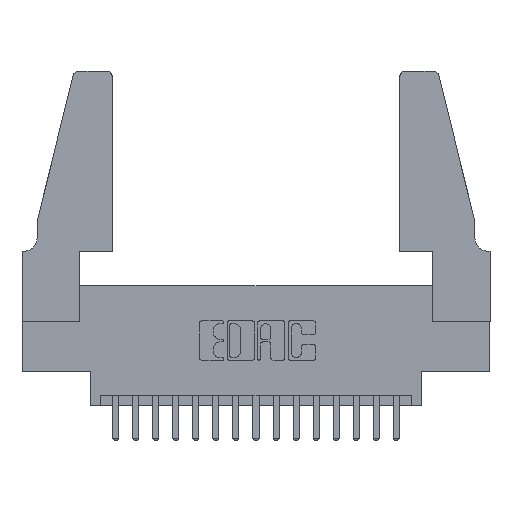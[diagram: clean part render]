
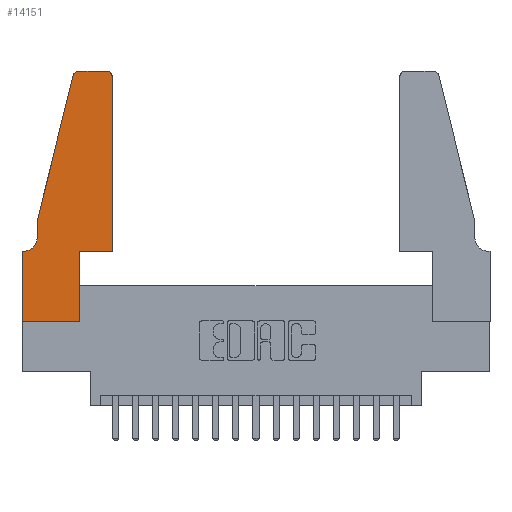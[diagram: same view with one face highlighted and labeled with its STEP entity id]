
A CAD part, top view. The second image highlights one B-rep face of the part: STEP entity #14151.
In plain terms, the highlighted planar face has unit normal (0, 0, 1).
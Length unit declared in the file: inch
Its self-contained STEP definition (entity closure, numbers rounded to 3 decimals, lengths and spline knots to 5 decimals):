
#932 = CARTESIAN_POINT ( 'NONE',  ( 0.284, 1.22, 0.37 ) ) ;
#951 = CARTESIAN_POINT ( 'NONE',  ( 0.2865, 0.35, 0.37 ) ) ;
#1338 = CARTESIAN_POINT ( 'NONE',  ( 0., 0.35, 0.37 ) ) ;
#1482 = ORIENTED_EDGE ( 'NONE', *, *, #4598, .T. ) ;
#1539 = ORIENTED_EDGE ( 'NONE', *, *, #6474, .T. ) ;
#1820 = EDGE_CURVE ( 'NONE', #3520, #6203, #15806, .T. ) ;
#2214 = CARTESIAN_POINT ( 'NONE',  ( 0.0055, 0.35, 0.37 ) ) ;
#2514 = LINE ( 'NONE', #17220, #11387 ) ;
#2531 = CIRCLE ( 'NONE', #7025, 0.03 ) ;
#2632 = CARTESIAN_POINT ( 'NONE',  ( 0.2605, 1.25, 0.37 ) ) ;
#2662 = ORIENTED_EDGE ( 'NONE', *, *, #1820, .T. ) ;
#2804 = CARTESIAN_POINT ( 'NONE',  ( 0., 0., 0.37 ) ) ;
#3079 = CARTESIAN_POINT ( 'NONE',  ( 0.25487, 1.22718, 0.37 ) ) ;
#3207 = CARTESIAN_POINT ( 'NONE',  ( 0.0755, 0.5, 0.37 ) ) ;
#3363 = VECTOR ( 'NONE', #14885, 39.37008 ) ;
#3466 = EDGE_CURVE ( 'NONE', #7415, #10062, #8599, .T. ) ;
#3520 = VERTEX_POINT ( 'NONE', #3079 ) ;
#3537 = DIRECTION ( 'NONE',  ( 1., 0., 0. ) ) ;
#3798 = VECTOR ( 'NONE', #5744, 39.37008 ) ;
#3944 = EDGE_CURVE ( 'NONE', #6162, #8397, #2531, .T. ) ;
#4045 = ORIENTED_EDGE ( 'NONE', *, *, #14664, .T. ) ;
#4072 = DIRECTION ( 'NONE',  ( 1., 0., 0. ) ) ;
#4356 = VECTOR ( 'NONE', #4590, 39.37008 ) ;
#4446 = LINE ( 'NONE', #15272, #3798 ) ;
#4590 = DIRECTION ( 'NONE',  ( -0.239, -0.971, 0. ) ) ;
#4598 = EDGE_CURVE ( 'NONE', #6203, #7415, #2514, .T. ) ;
#4744 = VERTEX_POINT ( 'NONE', #10787 ) ;
#4917 = DIRECTION ( 'NONE',  ( 0., 0., 1. ) ) ;
#5021 = EDGE_CURVE ( 'NONE', #13518, #6726, #4446, .T. ) ;
#5106 = VECTOR ( 'NONE', #7764, 39.37008 ) ;
#5264 = CARTESIAN_POINT ( 'NONE',  ( 0., 0.35, 0.37 ) ) ;
#5430 = CARTESIAN_POINT ( 'NONE',  ( 0., 0., 0.37 ) ) ;
#5569 = PLANE ( 'NONE',  #6043 ) ;
#5598 = CARTESIAN_POINT ( 'NONE',  ( 0.4205, 1.22, 0.37 ) ) ;
#5744 = DIRECTION ( 'NONE',  ( 0., -1., 0. ) ) ;
#5765 = LINE ( 'NONE', #2632, #3363 ) ;
#6043 = AXIS2_PLACEMENT_3D ( 'NONE', #1338, #11003, #7005 ) ;
#6162 = VERTEX_POINT ( 'NONE', #16697 ) ;
#6203 = VERTEX_POINT ( 'NONE', #9713 ) ;
#6394 = VERTEX_POINT ( 'NONE', #8518 ) ;
#6474 = EDGE_CURVE ( 'NONE', #10062, #13518, #8807, .T. ) ;
#6726 = VERTEX_POINT ( 'NONE', #2804 ) ;
#7005 = DIRECTION ( 'NONE',  ( 1., 0., 0. ) ) ;
#7025 = AXIS2_PLACEMENT_3D ( 'NONE', #5598, #8470, #4072 ) ;
#7278 = EDGE_CURVE ( 'NONE', #6394, #3520, #7693, .T. ) ;
#7415 = VERTEX_POINT ( 'NONE', #9623 ) ;
#7693 = CIRCLE ( 'NONE', #10425, 0.03 ) ;
#7754 = DIRECTION ( 'NONE',  ( 0., -1., 0. ) ) ;
#7764 = DIRECTION ( 'NONE',  ( 0., 1., 0. ) ) ;
#7924 = VECTOR ( 'NONE', #9757, 39.37008 ) ;
#8012 = VECTOR ( 'NONE', #15147, 39.37008 ) ;
#8107 = EDGE_CURVE ( 'NONE', #8888, #6162, #13905, .T. ) ;
#8397 = VERTEX_POINT ( 'NONE', #10443 ) ;
#8470 = DIRECTION ( 'NONE',  ( 0., 0., 1. ) ) ;
#8518 = CARTESIAN_POINT ( 'NONE',  ( 0.284, 1.25, 0.37 ) ) ;
#8599 = CIRCLE ( 'NONE', #16025, 0.07 ) ;
#8635 = VECTOR ( 'NONE', #3537, 39.37008 ) ;
#8807 = LINE ( 'NONE', #12284, #7924 ) ;
#8888 = VERTEX_POINT ( 'NONE', #11468 ) ;
#9009 = ORIENTED_EDGE ( 'NONE', *, *, #3466, .T. ) ;
#9128 = EDGE_LOOP ( 'NONE', ( #4045, #15290, #2662, #1482, #9009, #1539, #9952, #10769, #9778, #14565, #13995, #10145 ) ) ;
#9606 = EDGE_CURVE ( 'NONE', #6726, #4744, #13627, .T. ) ;
#9623 = CARTESIAN_POINT ( 'NONE',  ( 0.0755, 0.42, 0.37 ) ) ;
#9713 = CARTESIAN_POINT ( 'NONE',  ( 0.0755, 0.5, 0.37 ) ) ;
#9757 = DIRECTION ( 'NONE',  ( -1., 0., 0. ) ) ;
#9778 = ORIENTED_EDGE ( 'NONE', *, *, #14575, .T. ) ;
#9952 = ORIENTED_EDGE ( 'NONE', *, *, #5021, .T. ) ;
#10062 = VERTEX_POINT ( 'NONE', #2214 ) ;
#10145 = ORIENTED_EDGE ( 'NONE', *, *, #3944, .T. ) ;
#10308 = LINE ( 'NONE', #17454, #5106 ) ;
#10425 = AXIS2_PLACEMENT_3D ( 'NONE', #932, #4917, #15897 ) ;
#10443 = CARTESIAN_POINT ( 'NONE',  ( 0.4205, 1.25, 0.37 ) ) ;
#10769 = ORIENTED_EDGE ( 'NONE', *, *, #9606, .T. ) ;
#10787 = CARTESIAN_POINT ( 'NONE',  ( 0.2865, 0., 0.37 ) ) ;
#11003 = DIRECTION ( 'NONE',  ( 0., 0., 1. ) ) ;
#11387 = VECTOR ( 'NONE', #7754, 39.37008 ) ;
#11468 = CARTESIAN_POINT ( 'NONE',  ( 0.4505, 0.35, 0.37 ) ) ;
#12284 = CARTESIAN_POINT ( 'NONE',  ( 0.0755, 0.35, 0.37 ) ) ;
#12427 = DIRECTION ( 'NONE',  ( 0., 1., 0. ) ) ;
#12665 = EDGE_CURVE ( 'NONE', #12835, #8888, #12956, .T. ) ;
#12835 = VERTEX_POINT ( 'NONE', #951 ) ;
#12847 = VECTOR ( 'NONE', #12427, 39.37008 ) ;
#12956 = LINE ( 'NONE', #14394, #8635 ) ;
#13518 = VERTEX_POINT ( 'NONE', #5264 ) ;
#13627 = LINE ( 'NONE', #5430, #8012 ) ;
#13905 = LINE ( 'NONE', #16632, #12847 ) ;
#13955 = FACE_OUTER_BOUND ( 'NONE', #9128, .T. ) ;
#13995 = ORIENTED_EDGE ( 'NONE', *, *, #8107, .T. ) ;
#14052 = DIRECTION ( 'NONE',  ( 0., 0., -1. ) ) ;
#14151 = ADVANCED_FACE ( 'NONE', ( #13955 ), #5569, .T. ) ;
#14394 = CARTESIAN_POINT ( 'NONE',  ( 0.4505, 0.35, 0.37 ) ) ;
#14565 = ORIENTED_EDGE ( 'NONE', *, *, #12665, .T. ) ;
#14575 = EDGE_CURVE ( 'NONE', #4744, #12835, #10308, .T. ) ;
#14664 = EDGE_CURVE ( 'NONE', #8397, #6394, #5765, .T. ) ;
#14885 = DIRECTION ( 'NONE',  ( -1., 0., 0. ) ) ;
#15147 = DIRECTION ( 'NONE',  ( 1., 0., 0. ) ) ;
#15272 = CARTESIAN_POINT ( 'NONE',  ( 0., 0., 0.37 ) ) ;
#15290 = ORIENTED_EDGE ( 'NONE', *, *, #7278, .T. ) ;
#15408 = CARTESIAN_POINT ( 'NONE',  ( 0.0055, 0.42, 0.37 ) ) ;
#15806 = LINE ( 'NONE', #3207, #4356 ) ;
#15897 = DIRECTION ( 'NONE',  ( 1., 0., 0. ) ) ;
#16025 = AXIS2_PLACEMENT_3D ( 'NONE', #15408, #14052, #16886 ) ;
#16632 = CARTESIAN_POINT ( 'NONE',  ( 0.4505, 0.35, 0.37 ) ) ;
#16697 = CARTESIAN_POINT ( 'NONE',  ( 0.4505, 1.22, 0.37 ) ) ;
#16886 = DIRECTION ( 'NONE',  ( -1., 0., 0. ) ) ;
#17220 = CARTESIAN_POINT ( 'NONE',  ( 0.0755, 0.5, 0.37 ) ) ;
#17454 = CARTESIAN_POINT ( 'NONE',  ( 0.2865, 0.35, 0.37 ) ) ;
